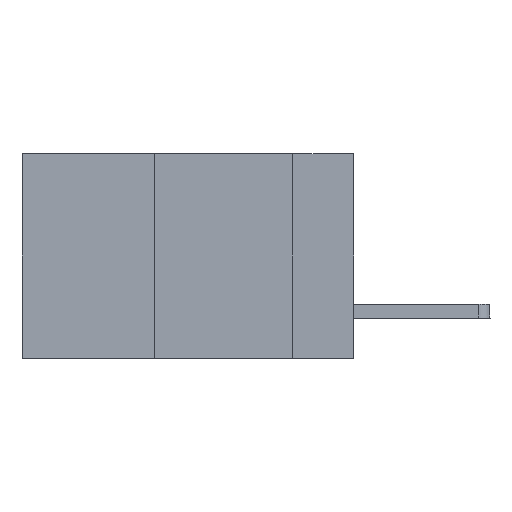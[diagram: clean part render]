
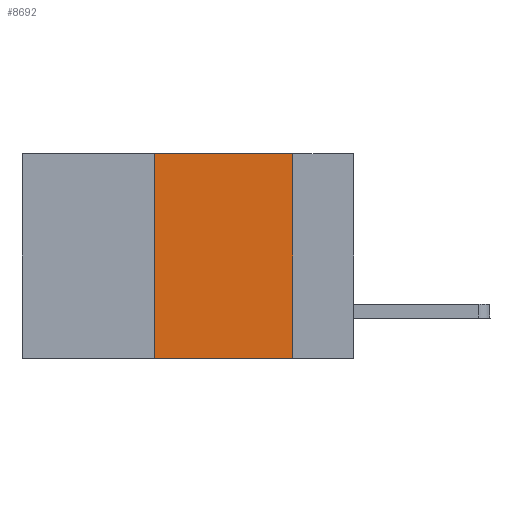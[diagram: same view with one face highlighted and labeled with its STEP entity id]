
A CAD part, left-side view. The second image highlights one B-rep face of the part: STEP entity #8692.
In plain terms, the highlighted planar face has unit normal (-1, 0, 0).
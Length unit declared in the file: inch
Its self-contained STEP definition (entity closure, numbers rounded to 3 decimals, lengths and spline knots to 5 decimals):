
#370 = VERTEX_POINT ( 'NONE', #3319 ) ;
#1218 = VERTEX_POINT ( 'NONE', #9363 ) ;
#1248 = LINE ( 'NONE', #10529, #3073 ) ;
#1907 = DIRECTION ( 'NONE',  ( 0., -1., 0. ) ) ;
#2387 = CARTESIAN_POINT ( 'NONE',  ( 0., 0.36, 0. ) ) ;
#2588 = ORIENTED_EDGE ( 'NONE', *, *, #10014, .F. ) ;
#2903 = CARTESIAN_POINT ( 'NONE',  ( 0., 0.6, 0. ) ) ;
#2997 = DIRECTION ( 'NONE',  ( 0., 0., -1. ) ) ;
#3073 = VECTOR ( 'NONE', #2997, 39.37008 ) ;
#3301 = DIRECTION ( 'NONE',  ( 0., -1., 0. ) ) ;
#3319 = CARTESIAN_POINT ( 'NONE',  ( 0., 0.11, 0. ) ) ;
#3815 = CARTESIAN_POINT ( 'NONE',  ( 0., 0.6, 0. ) ) ;
#3855 = LINE ( 'NONE', #6292, #9782 ) ;
#3913 = ORIENTED_EDGE ( 'NONE', *, *, #7532, .F. ) ;
#4305 = LINE ( 'NONE', #2903, #9595 ) ;
#4502 = AXIS2_PLACEMENT_3D ( 'NONE', #3815, #9018, #6039 ) ;
#4798 = EDGE_LOOP ( 'NONE', ( #2588, #8673, #3913, #5324 ) ) ;
#5324 = ORIENTED_EDGE ( 'NONE', *, *, #12218, .T. ) ;
#5945 = PLANE ( 'NONE',  #4502 ) ;
#6039 = DIRECTION ( 'NONE',  ( 0., 0., -1. ) ) ;
#6076 = CARTESIAN_POINT ( 'NONE',  ( 0., 0.11, -0.37 ) ) ;
#6292 = CARTESIAN_POINT ( 'NONE',  ( 0., 0.6, -0.37 ) ) ;
#6731 = DIRECTION ( 'NONE',  ( 0., 0., 1. ) ) ;
#7532 = EDGE_CURVE ( 'NONE', #13210, #1218, #11238, .T. ) ;
#7737 = FACE_OUTER_BOUND ( 'NONE', #4798, .T. ) ;
#7934 = VECTOR ( 'NONE', #6731, 39.37008 ) ;
#8497 = CARTESIAN_POINT ( 'NONE',  ( 0., 0.36, -0.37 ) ) ;
#8673 = ORIENTED_EDGE ( 'NONE', *, *, #12741, .F. ) ;
#8692 = ADVANCED_FACE ( 'NONE', ( #7737 ), #5945, .F. ) ;
#9018 = DIRECTION ( 'NONE',  ( 1., 0., 0. ) ) ;
#9363 = CARTESIAN_POINT ( 'NONE',  ( 0., 0.36, 0. ) ) ;
#9595 = VECTOR ( 'NONE', #1907, 39.37008 ) ;
#9782 = VECTOR ( 'NONE', #3301, 39.37008 ) ;
#10014 = EDGE_CURVE ( 'NONE', #370, #12706, #1248, .T. ) ;
#10529 = CARTESIAN_POINT ( 'NONE',  ( 0., 0.11, 0. ) ) ;
#11238 = LINE ( 'NONE', #2387, #7934 ) ;
#12218 = EDGE_CURVE ( 'NONE', #13210, #12706, #3855, .T. ) ;
#12706 = VERTEX_POINT ( 'NONE', #6076 ) ;
#12741 = EDGE_CURVE ( 'NONE', #1218, #370, #4305, .T. ) ;
#13210 = VERTEX_POINT ( 'NONE', #8497 ) ;
